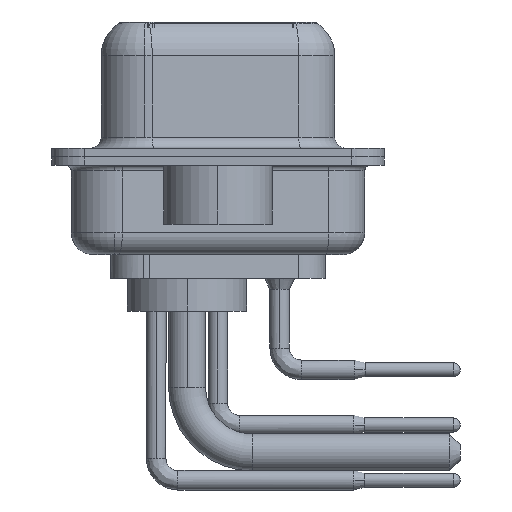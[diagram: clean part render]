
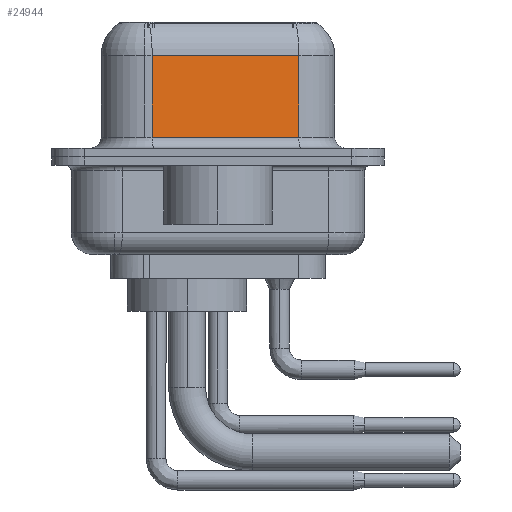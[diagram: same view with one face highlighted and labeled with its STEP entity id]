
A CAD part, left-side view. The second image highlights one B-rep face of the part: STEP entity #24944.
In plain terms, the highlighted planar face has unit normal (-0.985, -0.174, 0).
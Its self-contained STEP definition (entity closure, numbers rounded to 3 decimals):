
#278 = ORIENTED_EDGE ( 'NONE', *, *, #26438, .T. ) ;
#1466 = CARTESIAN_POINT ( 'NONE',  ( 5.621, -3.722, 0.9 ) ) ;
#1546 = EDGE_CURVE ( 'NONE', #5150, #13086, #21654, .T. ) ;
#2714 = CARTESIAN_POINT ( 'NONE',  ( 5.621, -3.722, 6.4 ) ) ;
#3496 = VERTEX_POINT ( 'NONE', #14051 ) ;
#5150 = VERTEX_POINT ( 'NONE', #21043 ) ;
#5487 = CARTESIAN_POINT ( 'NONE',  ( 4.43, 3.028, 0.9 ) ) ;
#5977 = DIRECTION ( 'NONE',  ( 0., 0., -1. ) ) ;
#6403 = CARTESIAN_POINT ( 'NONE',  ( 4.43, 3.028, 6.4 ) ) ;
#8623 = EDGE_LOOP ( 'NONE', ( #11078, #12200, #278, #14713 ) ) ;
#10951 = VECTOR ( 'NONE', #17418, 1000. ) ;
#11078 = ORIENTED_EDGE ( 'NONE', *, *, #1546, .F. ) ;
#11657 = DIRECTION ( 'NONE',  ( -0.174, 0.985, 0. ) ) ;
#12200 = ORIENTED_EDGE ( 'NONE', *, *, #18286, .T. ) ;
#12416 = VERTEX_POINT ( 'NONE', #5487 ) ;
#13086 = VERTEX_POINT ( 'NONE', #1466 ) ;
#14051 = CARTESIAN_POINT ( 'NONE',  ( 4.43, 3.028, 4.65 ) ) ;
#14055 = AXIS2_PLACEMENT_3D ( 'NONE', #2714, #22900, #11657 ) ;
#14713 = ORIENTED_EDGE ( 'NONE', *, *, #23959, .T. ) ;
#15131 = DIRECTION ( 'NONE',  ( 0., 0., -1. ) ) ;
#15188 = LINE ( 'NONE', #16836, #10951 ) ;
#15870 = LINE ( 'NONE', #24895, #27233 ) ;
#16836 = CARTESIAN_POINT ( 'NONE',  ( 5.621, -3.722, 4.65 ) ) ;
#17418 = DIRECTION ( 'NONE',  ( -0.174, 0.985, 0. ) ) ;
#18286 = EDGE_CURVE ( 'NONE', #5150, #3496, #15188, .T. ) ;
#19933 = LINE ( 'NONE', #6403, #21730 ) ;
#20465 = DIRECTION ( 'NONE',  ( 0.174, -0.985, 0. ) ) ;
#20681 = PLANE ( 'NONE',  #14055 ) ;
#21043 = CARTESIAN_POINT ( 'NONE',  ( 5.621, -3.722, 4.65 ) ) ;
#21654 = LINE ( 'NONE', #23728, #26182 ) ;
#21730 = VECTOR ( 'NONE', #5977, 1000. ) ;
#22900 = DIRECTION ( 'NONE',  ( 0.985, 0.174, 0. ) ) ;
#23040 = FACE_OUTER_BOUND ( 'NONE', #8623, .T. ) ;
#23728 = CARTESIAN_POINT ( 'NONE',  ( 5.621, -3.722, 6.4 ) ) ;
#23959 = EDGE_CURVE ( 'NONE', #12416, #13086, #15870, .T. ) ;
#24895 = CARTESIAN_POINT ( 'NONE',  ( 5.621, -3.722, 0.9 ) ) ;
#24944 = ADVANCED_FACE ( 'NONE', ( #23040 ), #20681, .F. ) ;
#26182 = VECTOR ( 'NONE', #15131, 1000. ) ;
#26438 = EDGE_CURVE ( 'NONE', #3496, #12416, #19933, .T. ) ;
#27233 = VECTOR ( 'NONE', #20465, 1000. ) ;
